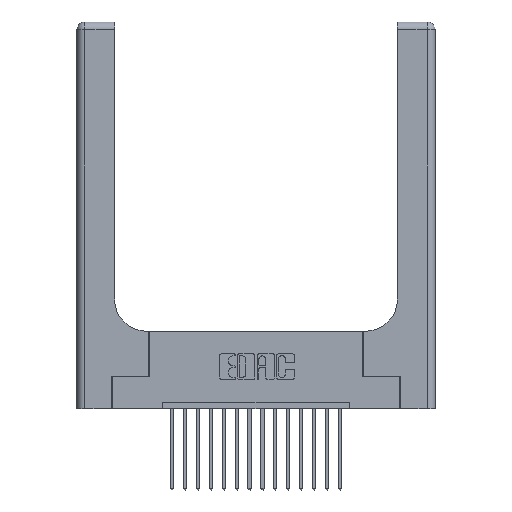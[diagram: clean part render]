
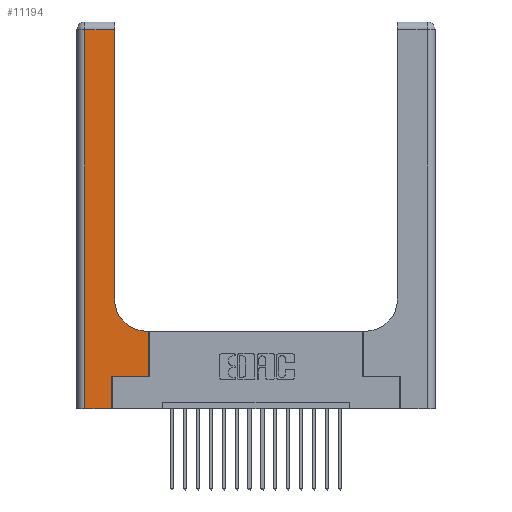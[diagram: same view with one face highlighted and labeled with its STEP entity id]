
A CAD part, top view. The second image highlights one B-rep face of the part: STEP entity #11194.
In plain terms, the highlighted planar face has unit normal (0, 0, 1).
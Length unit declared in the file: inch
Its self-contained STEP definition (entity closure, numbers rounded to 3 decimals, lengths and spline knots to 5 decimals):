
#225 = VECTOR ( 'NONE', #5840, 39.37008 ) ;
#875 = ORIENTED_EDGE ( 'NONE', *, *, #5318, .T. ) ;
#902 = DIRECTION ( 'NONE',  ( -1., 0., 0. ) ) ;
#1010 = DIRECTION ( 'NONE',  ( 0., 0., -1. ) ) ;
#2093 = LINE ( 'NONE', #17775, #9126 ) ;
#2940 = DIRECTION ( 'NONE',  ( -1., 0., 0. ) ) ;
#3493 = EDGE_LOOP ( 'NONE', ( #7330, #875, #12860, #15574, #9717, #12534, #14185, #8238, #6231 ) ) ;
#3665 = CARTESIAN_POINT ( 'NONE',  ( 0.5585, 0.6, 0.37 ) ) ;
#4441 = EDGE_CURVE ( 'NONE', #13614, #6164, #15183, .T. ) ;
#5152 = LINE ( 'NONE', #15047, #225 ) ;
#5180 = EDGE_CURVE ( 'NONE', #6164, #16631, #12049, .T. ) ;
#5318 = EDGE_CURVE ( 'NONE', #8115, #13303, #8994, .T. ) ;
#5548 = VERTEX_POINT ( 'NONE', #18952 ) ;
#5840 = DIRECTION ( 'NONE',  ( 0., 1., 0. ) ) ;
#6164 = VERTEX_POINT ( 'NONE', #8516 ) ;
#6231 = ORIENTED_EDGE ( 'NONE', *, *, #6609, .T. ) ;
#6244 = DIRECTION ( 'NONE',  ( 0., 1., 0. ) ) ;
#6485 = CARTESIAN_POINT ( 'NONE',  ( 0.2915, 2.94, 0.37 ) ) ;
#6609 = EDGE_CURVE ( 'NONE', #19270, #11507, #10850, .T. ) ;
#6800 = CARTESIAN_POINT ( 'NONE',  ( 0.2915, 0.6, 0.37 ) ) ;
#6882 = VECTOR ( 'NONE', #12344, 39.37008 ) ;
#7330 = ORIENTED_EDGE ( 'NONE', *, *, #15455, .T. ) ;
#7411 = VECTOR ( 'NONE', #18853, 39.37008 ) ;
#7611 = VECTOR ( 'NONE', #902, 39.37008 ) ;
#7863 = CARTESIAN_POINT ( 'NONE',  ( 0., 2.94, 0.37 ) ) ;
#8115 = VERTEX_POINT ( 'NONE', #6485 ) ;
#8124 = CARTESIAN_POINT ( 'NONE',  ( 0.269, 0.25, 0.37 ) ) ;
#8238 = ORIENTED_EDGE ( 'NONE', *, *, #19392, .T. ) ;
#8489 = EDGE_CURVE ( 'NONE', #5548, #13614, #5152, .T. ) ;
#8516 = CARTESIAN_POINT ( 'NONE',  ( 0.5585, 0.25, 0.37 ) ) ;
#8910 = PLANE ( 'NONE',  #12126 ) ;
#8994 = LINE ( 'NONE', #7863, #6882 ) ;
#9126 = VECTOR ( 'NONE', #11678, 39.37008 ) ;
#9716 = FACE_OUTER_BOUND ( 'NONE', #3493, .T. ) ;
#9717 = ORIENTED_EDGE ( 'NONE', *, *, #8489, .T. ) ;
#9960 = CARTESIAN_POINT ( 'NONE',  ( 0.06, 2.94, 0.37 ) ) ;
#10127 = CARTESIAN_POINT ( 'NONE',  ( 0.06, 0., 0.37 ) ) ;
#10574 = CARTESIAN_POINT ( 'NONE',  ( 0.2915, 0.85, 0.37 ) ) ;
#10638 = VECTOR ( 'NONE', #6244, 39.37008 ) ;
#10850 = CIRCLE ( 'NONE', #19389, 0.25 ) ;
#11194 = ADVANCED_FACE ( 'NONE', ( #9716 ), #8910, .F. ) ;
#11315 = DIRECTION ( 'NONE',  ( 1., 0., 0. ) ) ;
#11507 = VERTEX_POINT ( 'NONE', #10574 ) ;
#11678 = DIRECTION ( 'NONE',  ( 0., -1., 0. ) ) ;
#11928 = CARTESIAN_POINT ( 'NONE',  ( 0., 3., 0.37 ) ) ;
#12049 = LINE ( 'NONE', #15268, #10638 ) ;
#12126 = AXIS2_PLACEMENT_3D ( 'NONE', #11928, #13458, #2940 ) ;
#12344 = DIRECTION ( 'NONE',  ( -1., 0., 0. ) ) ;
#12534 = ORIENTED_EDGE ( 'NONE', *, *, #4441, .T. ) ;
#12814 = CARTESIAN_POINT ( 'NONE',  ( 0., 0., 0.37 ) ) ;
#12860 = ORIENTED_EDGE ( 'NONE', *, *, #16332, .T. ) ;
#12960 = CARTESIAN_POINT ( 'NONE',  ( 0.5415, 0.85, 0.37 ) ) ;
#13041 = DIRECTION ( 'NONE',  ( 0., 1., 0. ) ) ;
#13303 = VERTEX_POINT ( 'NONE', #9960 ) ;
#13458 = DIRECTION ( 'NONE',  ( 0., 0., -1. ) ) ;
#13614 = VERTEX_POINT ( 'NONE', #8124 ) ;
#13929 = VERTEX_POINT ( 'NONE', #10127 ) ;
#14185 = ORIENTED_EDGE ( 'NONE', *, *, #5180, .T. ) ;
#14934 = VECTOR ( 'NONE', #16045, 39.37008 ) ;
#14990 = LINE ( 'NONE', #12814, #7411 ) ;
#15047 = CARTESIAN_POINT ( 'NONE',  ( 0.269, 0., 0.37 ) ) ;
#15183 = LINE ( 'NONE', #17524, #14934 ) ;
#15268 = CARTESIAN_POINT ( 'NONE',  ( 0.5585, 0.25, 0.37 ) ) ;
#15455 = EDGE_CURVE ( 'NONE', #11507, #8115, #19518, .T. ) ;
#15574 = ORIENTED_EDGE ( 'NONE', *, *, #17729, .T. ) ;
#16045 = DIRECTION ( 'NONE',  ( 1., 0., 0. ) ) ;
#16332 = EDGE_CURVE ( 'NONE', #13303, #13929, #2093, .T. ) ;
#16631 = VERTEX_POINT ( 'NONE', #3665 ) ;
#16902 = CARTESIAN_POINT ( 'NONE',  ( 0.5415, 0.6, 0.37 ) ) ;
#16917 = VECTOR ( 'NONE', #13041, 39.37008 ) ;
#17524 = CARTESIAN_POINT ( 'NONE',  ( 0.269, 0.25, 0.37 ) ) ;
#17729 = EDGE_CURVE ( 'NONE', #13929, #5548, #14990, .T. ) ;
#17775 = CARTESIAN_POINT ( 'NONE',  ( 0.06, 3., 0.37 ) ) ;
#18853 = DIRECTION ( 'NONE',  ( 1., 0., 0. ) ) ;
#18952 = CARTESIAN_POINT ( 'NONE',  ( 0.269, 0., 0.37 ) ) ;
#19078 = CARTESIAN_POINT ( 'NONE',  ( 0.2915, 3., 0.37 ) ) ;
#19204 = LINE ( 'NONE', #6800, #7611 ) ;
#19270 = VERTEX_POINT ( 'NONE', #16902 ) ;
#19389 = AXIS2_PLACEMENT_3D ( 'NONE', #12960, #1010, #11315 ) ;
#19392 = EDGE_CURVE ( 'NONE', #16631, #19270, #19204, .T. ) ;
#19518 = LINE ( 'NONE', #19078, #16917 ) ;
